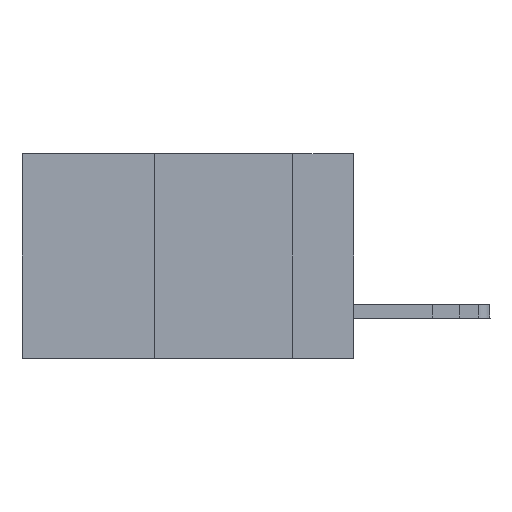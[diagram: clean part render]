
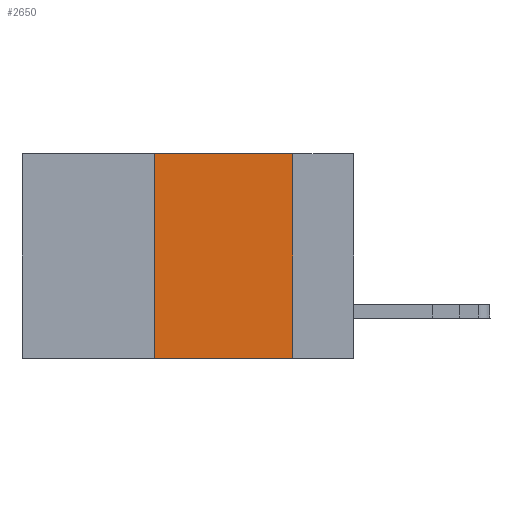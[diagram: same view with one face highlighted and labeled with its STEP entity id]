
A CAD part, left-side view. The second image highlights one B-rep face of the part: STEP entity #2650.
In plain terms, the highlighted planar face has unit normal (-1, 0, 0).
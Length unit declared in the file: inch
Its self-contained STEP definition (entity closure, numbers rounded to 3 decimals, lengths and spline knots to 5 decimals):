
#2650 = ADVANCED_FACE ( 'NONE', ( #27256 ), #24481, .F. ) ;
#3269 = CARTESIAN_POINT ( 'NONE',  ( 0., 0.6, 0. ) ) ;
#3626 = DIRECTION ( 'NONE',  ( 0., 0., -1. ) ) ;
#5265 = VERTEX_POINT ( 'NONE', #30252 ) ;
#6314 = VERTEX_POINT ( 'NONE', #14632 ) ;
#6802 = ORIENTED_EDGE ( 'NONE', *, *, #31879, .F. ) ;
#7839 = DIRECTION ( 'NONE',  ( 0., -1., 0. ) ) ;
#11904 = ORIENTED_EDGE ( 'NONE', *, *, #13311, .T. ) ;
#12010 = EDGE_LOOP ( 'NONE', ( #26001, #6802, #15692, #11904 ) ) ;
#12068 = EDGE_CURVE ( 'NONE', #17477, #6314, #15007, .T. ) ;
#12157 = CARTESIAN_POINT ( 'NONE',  ( 0., 0.36, 0. ) ) ;
#12382 = LINE ( 'NONE', #29985, #13998 ) ;
#13311 = EDGE_CURVE ( 'NONE', #16874, #6314, #28309, .T. ) ;
#13803 = DIRECTION ( 'NONE',  ( 1., 0., 0. ) ) ;
#13998 = VECTOR ( 'NONE', #7839, 39.37008 ) ;
#14399 = DIRECTION ( 'NONE',  ( 0., 0., 1. ) ) ;
#14578 = EDGE_CURVE ( 'NONE', #16874, #5265, #17467, .T. ) ;
#14632 = CARTESIAN_POINT ( 'NONE',  ( 0., 0.11, -0.37 ) ) ;
#14698 = DIRECTION ( 'NONE',  ( 0., -1., 0. ) ) ;
#15007 = LINE ( 'NONE', #17236, #33769 ) ;
#15692 = ORIENTED_EDGE ( 'NONE', *, *, #14578, .F. ) ;
#16874 = VERTEX_POINT ( 'NONE', #24789 ) ;
#17236 = CARTESIAN_POINT ( 'NONE',  ( 0., 0.11, 0. ) ) ;
#17467 = LINE ( 'NONE', #12157, #22272 ) ;
#17477 = VERTEX_POINT ( 'NONE', #23628 ) ;
#19678 = AXIS2_PLACEMENT_3D ( 'NONE', #3269, #13803, #3626 ) ;
#20169 = CARTESIAN_POINT ( 'NONE',  ( 0., 0.6, -0.37 ) ) ;
#22272 = VECTOR ( 'NONE', #14399, 39.37008 ) ;
#23287 = VECTOR ( 'NONE', #14698, 39.37008 ) ;
#23628 = CARTESIAN_POINT ( 'NONE',  ( 0., 0.11, 0. ) ) ;
#24481 = PLANE ( 'NONE',  #19678 ) ;
#24789 = CARTESIAN_POINT ( 'NONE',  ( 0., 0.36, -0.37 ) ) ;
#26001 = ORIENTED_EDGE ( 'NONE', *, *, #12068, .F. ) ;
#27256 = FACE_OUTER_BOUND ( 'NONE', #12010, .T. ) ;
#27805 = DIRECTION ( 'NONE',  ( 0., 0., -1. ) ) ;
#28309 = LINE ( 'NONE', #20169, #23287 ) ;
#29985 = CARTESIAN_POINT ( 'NONE',  ( 0., 0.6, 0. ) ) ;
#30252 = CARTESIAN_POINT ( 'NONE',  ( 0., 0.36, 0. ) ) ;
#31879 = EDGE_CURVE ( 'NONE', #5265, #17477, #12382, .T. ) ;
#33769 = VECTOR ( 'NONE', #27805, 39.37008 ) ;
